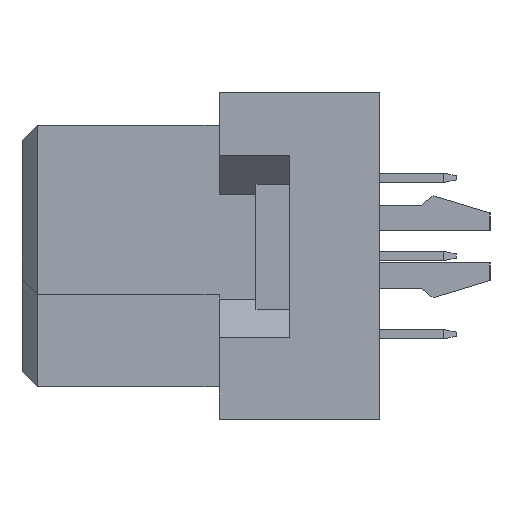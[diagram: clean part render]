
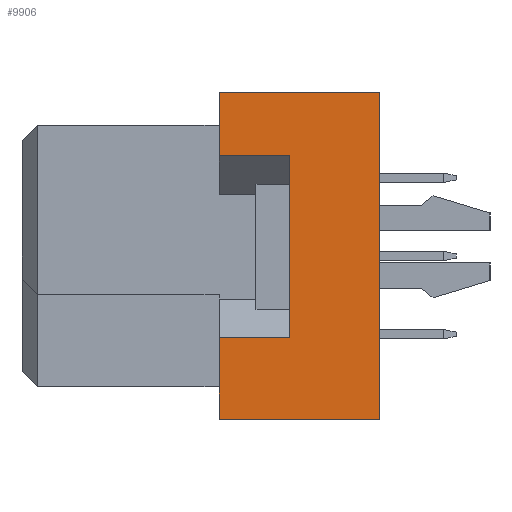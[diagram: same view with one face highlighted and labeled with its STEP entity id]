
A CAD part, left-side view. The second image highlights one B-rep face of the part: STEP entity #9906.
In plain terms, the highlighted planar face has unit normal (-1, 0, 0).
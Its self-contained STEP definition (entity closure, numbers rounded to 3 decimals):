
#36 = ORIENTED_EDGE ( 'NONE', *, *, #40859, .F. ) ;
#111 = DIRECTION ( 'NONE',  ( 0., 0., 1. ) ) ;
#462 = CARTESIAN_POINT ( 'NONE',  ( -47.5, -8.7, 3.25 ) ) ;
#1221 = DIRECTION ( 'NONE',  ( 0., 0., 1. ) ) ;
#2095 = DIRECTION ( 'NONE',  ( 0., 0., 1. ) ) ;
#2203 = EDGE_CURVE ( 'NONE', #20413, #12327, #38622, .T. ) ;
#2512 = VERTEX_POINT ( 'NONE', #41099 ) ;
#3440 = VERTEX_POINT ( 'NONE', #11804 ) ;
#3669 = AXIS2_PLACEMENT_3D ( 'NONE', #18993, #31830, #111 ) ;
#3781 = DIRECTION ( 'NONE',  ( 0., 1., 0. ) ) ;
#4389 = DIRECTION ( 'NONE',  ( 0., 0., 1. ) ) ;
#5167 = VERTEX_POINT ( 'NONE', #18160 ) ;
#5245 = ORIENTED_EDGE ( 'NONE', *, *, #25181, .T. ) ;
#6204 = PLANE ( 'NONE',  #3669 ) ;
#7872 = ORIENTED_EDGE ( 'NONE', *, *, #39530, .F. ) ;
#8192 = CARTESIAN_POINT ( 'NONE',  ( -47.5, -6.4, -5.3 ) ) ;
#8674 = DIRECTION ( 'NONE',  ( 0., 1., 0. ) ) ;
#8900 = ORIENTED_EDGE ( 'NONE', *, *, #25338, .F. ) ;
#9906 = ADVANCED_FACE ( 'NONE', ( #38761 ), #6204, .T. ) ;
#10177 = VECTOR ( 'NONE', #8674, 1000. ) ;
#11804 = CARTESIAN_POINT ( 'NONE',  ( -47.5, -11.6, 5.3 ) ) ;
#12327 = VERTEX_POINT ( 'NONE', #34204 ) ;
#12366 = EDGE_LOOP ( 'NONE', ( #23512, #8900, #18713, #34430, #5245, #36, #7872, #27317 ) ) ;
#12598 = LINE ( 'NONE', #38233, #16239 ) ;
#13197 = DIRECTION ( 'NONE',  ( 0., 0., 1. ) ) ;
#13368 = VECTOR ( 'NONE', #16197, 1000. ) ;
#13887 = LINE ( 'NONE', #27065, #28048 ) ;
#14529 = VERTEX_POINT ( 'NONE', #35926 ) ;
#14683 = DIRECTION ( 'NONE',  ( 0., 1., 0. ) ) ;
#14909 = CARTESIAN_POINT ( 'NONE',  ( -47.5, -6.4, -2.65 ) ) ;
#14962 = CARTESIAN_POINT ( 'NONE',  ( -47.5, -8.7, -2.65 ) ) ;
#16197 = DIRECTION ( 'NONE',  ( 0., 1., 0. ) ) ;
#16239 = VECTOR ( 'NONE', #3781, 1000. ) ;
#17600 = VECTOR ( 'NONE', #2095, 1000. ) ;
#18160 = CARTESIAN_POINT ( 'NONE',  ( -47.5, -6.4, -5.3 ) ) ;
#18713 = ORIENTED_EDGE ( 'NONE', *, *, #38385, .F. ) ;
#18993 = CARTESIAN_POINT ( 'NONE',  ( -47.5, -11.6, 5.3 ) ) ;
#19758 = LINE ( 'NONE', #462, #13368 ) ;
#20413 = VERTEX_POINT ( 'NONE', #24153 ) ;
#20584 = VERTEX_POINT ( 'NONE', #14909 ) ;
#23512 = ORIENTED_EDGE ( 'NONE', *, *, #27503, .T. ) ;
#23898 = CARTESIAN_POINT ( 'NONE',  ( -47.5, -6.4, -5.3 ) ) ;
#24153 = CARTESIAN_POINT ( 'NONE',  ( -47.5, -8.7, -2.65 ) ) ;
#24208 = LINE ( 'NONE', #14962, #10177 ) ;
#25181 = EDGE_CURVE ( 'NONE', #3440, #2512, #12598, .T. ) ;
#25338 = EDGE_CURVE ( 'NONE', #5167, #20584, #33157, .T. ) ;
#27065 = CARTESIAN_POINT ( 'NONE',  ( -47.5, -11.6, -5.3 ) ) ;
#27317 = ORIENTED_EDGE ( 'NONE', *, *, #2203, .F. ) ;
#27503 = EDGE_CURVE ( 'NONE', #20413, #20584, #24208, .T. ) ;
#27709 = LINE ( 'NONE', #8192, #17600 ) ;
#28048 = VECTOR ( 'NONE', #14683, 1000. ) ;
#29293 = EDGE_CURVE ( 'NONE', #36202, #3440, #38407, .T. ) ;
#30057 = CARTESIAN_POINT ( 'NONE',  ( -47.5, -11.6, -5.3 ) ) ;
#31830 = DIRECTION ( 'NONE',  ( -1., 0., 0. ) ) ;
#32739 = CARTESIAN_POINT ( 'NONE',  ( -47.5, -8.7, -2.65 ) ) ;
#33157 = LINE ( 'NONE', #23898, #34300 ) ;
#34204 = CARTESIAN_POINT ( 'NONE',  ( -47.5, -8.7, 3.25 ) ) ;
#34300 = VECTOR ( 'NONE', #4389, 1000. ) ;
#34430 = ORIENTED_EDGE ( 'NONE', *, *, #29293, .T. ) ;
#34574 = VECTOR ( 'NONE', #1221, 1000. ) ;
#35926 = CARTESIAN_POINT ( 'NONE',  ( -47.5, -6.4, 3.25 ) ) ;
#36202 = VERTEX_POINT ( 'NONE', #30057 ) ;
#38233 = CARTESIAN_POINT ( 'NONE',  ( -47.5, -11.6, 5.3 ) ) ;
#38385 = EDGE_CURVE ( 'NONE', #36202, #5167, #13887, .T. ) ;
#38407 = LINE ( 'NONE', #38617, #38443 ) ;
#38443 = VECTOR ( 'NONE', #13197, 1000. ) ;
#38617 = CARTESIAN_POINT ( 'NONE',  ( -47.5, -11.6, 5.3 ) ) ;
#38622 = LINE ( 'NONE', #32739, #34574 ) ;
#38761 = FACE_OUTER_BOUND ( 'NONE', #12366, .T. ) ;
#39530 = EDGE_CURVE ( 'NONE', #12327, #14529, #19758, .T. ) ;
#40859 = EDGE_CURVE ( 'NONE', #14529, #2512, #27709, .T. ) ;
#41099 = CARTESIAN_POINT ( 'NONE',  ( -47.5, -6.4, 5.3 ) ) ;
